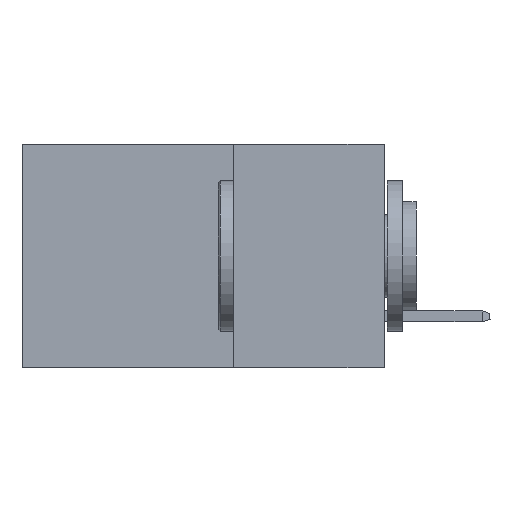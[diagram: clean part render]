
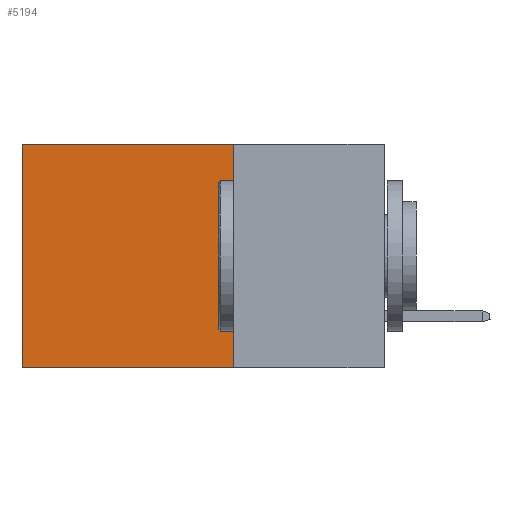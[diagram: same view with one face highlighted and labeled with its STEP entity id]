
A CAD part, left-side view. The second image highlights one B-rep face of the part: STEP entity #5194.
In plain terms, the highlighted planar face has unit normal (-1, 0, 0).
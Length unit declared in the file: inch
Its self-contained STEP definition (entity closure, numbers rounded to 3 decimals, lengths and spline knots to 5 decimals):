
#768 = EDGE_CURVE ( 'NONE', #10349, #24802, #4690, .T. ) ;
#1376 = CARTESIAN_POINT ( 'NONE',  ( 0.298, 0.6, 0. ) ) ;
#3061 = DIRECTION ( 'NONE',  ( 1., 0., 0. ) ) ;
#3553 = VECTOR ( 'NONE', #7701, 39.37008 ) ;
#4690 = LINE ( 'NONE', #13151, #21712 ) ;
#5194 = ADVANCED_FACE ( 'NONE', ( #12101 ), #12949, .F. ) ;
#6221 = EDGE_CURVE ( 'NONE', #24802, #10991, #24859, .T. ) ;
#6792 = EDGE_LOOP ( 'NONE', ( #14665, #19086, #8919, #25198 ) ) ;
#7671 = CARTESIAN_POINT ( 'NONE',  ( 0.298, 0.25, 0. ) ) ;
#7701 = DIRECTION ( 'NONE',  ( 0., 0., -1. ) ) ;
#8178 = CARTESIAN_POINT ( 'NONE',  ( 0.298, 0.25, 0. ) ) ;
#8919 = ORIENTED_EDGE ( 'NONE', *, *, #21502, .F. ) ;
#9700 = EDGE_CURVE ( 'NONE', #23434, #10991, #22509, .T. ) ;
#10229 = DIRECTION ( 'NONE',  ( 0., 0., -1. ) ) ;
#10349 = VERTEX_POINT ( 'NONE', #7671 ) ;
#10991 = VERTEX_POINT ( 'NONE', #12406 ) ;
#12101 = FACE_OUTER_BOUND ( 'NONE', #6792, .T. ) ;
#12168 = VECTOR ( 'NONE', #16303, 39.37008 ) ;
#12406 = CARTESIAN_POINT ( 'NONE',  ( 0.298, 0.6, -0.37 ) ) ;
#12949 = PLANE ( 'NONE',  #16132 ) ;
#13151 = CARTESIAN_POINT ( 'NONE',  ( 0.298, 0.25, 0. ) ) ;
#14162 = CARTESIAN_POINT ( 'NONE',  ( 0.298, 0.25, -0.37 ) ) ;
#14665 = ORIENTED_EDGE ( 'NONE', *, *, #6221, .T. ) ;
#14829 = DIRECTION ( 'NONE',  ( 0., 1., 0. ) ) ;
#14886 = CARTESIAN_POINT ( 'NONE',  ( 0.298, 0.25, 0. ) ) ;
#15253 = LINE ( 'NONE', #8178, #19786 ) ;
#15922 = CARTESIAN_POINT ( 'NONE',  ( 0.298, 0.6, 0. ) ) ;
#16132 = AXIS2_PLACEMENT_3D ( 'NONE', #14886, #3061, #22526 ) ;
#16303 = DIRECTION ( 'NONE',  ( 0., 1., 0. ) ) ;
#19086 = ORIENTED_EDGE ( 'NONE', *, *, #9700, .F. ) ;
#19786 = VECTOR ( 'NONE', #10229, 39.37008 ) ;
#21502 = EDGE_CURVE ( 'NONE', #10349, #23434, #15253, .T. ) ;
#21712 = VECTOR ( 'NONE', #14829, 39.37008 ) ;
#22244 = CARTESIAN_POINT ( 'NONE',  ( 0.298, 0.25, -0.37 ) ) ;
#22509 = LINE ( 'NONE', #14162, #12168 ) ;
#22526 = DIRECTION ( 'NONE',  ( 0., 0., -1. ) ) ;
#23434 = VERTEX_POINT ( 'NONE', #22244 ) ;
#24802 = VERTEX_POINT ( 'NONE', #15922 ) ;
#24859 = LINE ( 'NONE', #1376, #3553 ) ;
#25198 = ORIENTED_EDGE ( 'NONE', *, *, #768, .T. ) ;
